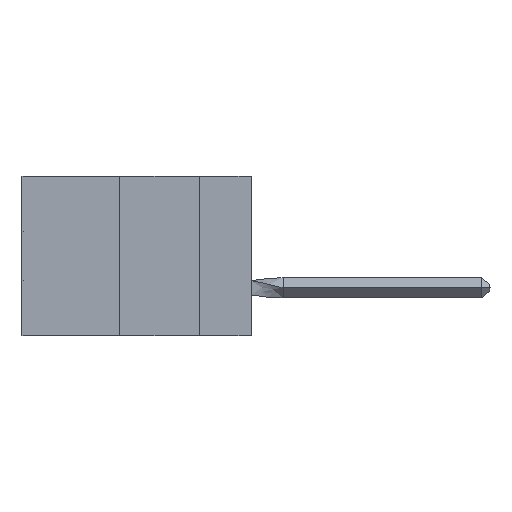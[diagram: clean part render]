
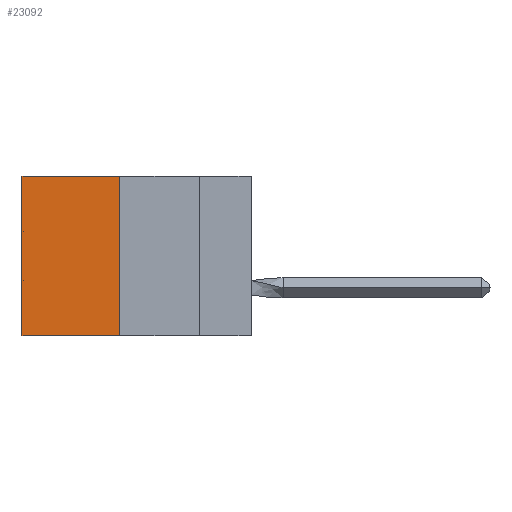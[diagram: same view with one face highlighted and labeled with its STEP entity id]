
A CAD part, left-side view. The second image highlights one B-rep face of the part: STEP entity #23092.
In plain terms, the highlighted planar face has unit normal (-1, 0, 0).
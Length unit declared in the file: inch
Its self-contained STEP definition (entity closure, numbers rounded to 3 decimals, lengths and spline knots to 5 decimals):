
#3802 = VECTOR ( 'NONE', #44119, 39.37008 ) ;
#6361 = VERTEX_POINT ( 'NONE', #9219 ) ;
#6470 = EDGE_CURVE ( 'NONE', #21489, #6361, #34841, .T. ) ;
#9219 = CARTESIAN_POINT ( 'NONE',  ( 0.305, 0.72, -0.5 ) ) ;
#9401 = EDGE_CURVE ( 'NONE', #30376, #21489, #21470, .T. ) ;
#9941 = FACE_OUTER_BOUND ( 'NONE', #44193, .T. ) ;
#12014 = DIRECTION ( 'NONE',  ( 0., 1., 0. ) ) ;
#12082 = VERTEX_POINT ( 'NONE', #38996 ) ;
#12298 = AXIS2_PLACEMENT_3D ( 'NONE', #26361, #12898, #33242 ) ;
#12898 = DIRECTION ( 'NONE',  ( 1., 0., 0. ) ) ;
#16788 = CARTESIAN_POINT ( 'NONE',  ( 0.305, 0.413, -0.5 ) ) ;
#17847 = ORIENTED_EDGE ( 'NONE', *, *, #36858, .T. ) ;
#18082 = CARTESIAN_POINT ( 'NONE',  ( 0.305, 0.413, 0. ) ) ;
#19926 = DIRECTION ( 'NONE',  ( 0., 0., -1. ) ) ;
#21470 = LINE ( 'NONE', #30815, #30567 ) ;
#21489 = VERTEX_POINT ( 'NONE', #39032 ) ;
#22206 = CARTESIAN_POINT ( 'NONE',  ( 0.305, 0.413, 0. ) ) ;
#23092 = ADVANCED_FACE ( 'NONE', ( #9941 ), #37121, .F. ) ;
#26361 = CARTESIAN_POINT ( 'NONE',  ( 0.305, 0.413, -0.5 ) ) ;
#27143 = ORIENTED_EDGE ( 'NONE', *, *, #35543, .T. ) ;
#27373 = LINE ( 'NONE', #22206, #38057 ) ;
#27498 = LINE ( 'NONE', #30596, #34481 ) ;
#28804 = ORIENTED_EDGE ( 'NONE', *, *, #9401, .F. ) ;
#30376 = VERTEX_POINT ( 'NONE', #18082 ) ;
#30567 = VECTOR ( 'NONE', #19926, 39.37008 ) ;
#30596 = CARTESIAN_POINT ( 'NONE',  ( 0.305, 0.72, -0.5 ) ) ;
#30815 = CARTESIAN_POINT ( 'NONE',  ( 0.305, 0.413, -0.5 ) ) ;
#33242 = DIRECTION ( 'NONE',  ( 0., 0., -1. ) ) ;
#34481 = VECTOR ( 'NONE', #43976, 39.37008 ) ;
#34539 = ORIENTED_EDGE ( 'NONE', *, *, #6470, .F. ) ;
#34841 = LINE ( 'NONE', #16788, #3802 ) ;
#35543 = EDGE_CURVE ( 'NONE', #12082, #6361, #27498, .T. ) ;
#36858 = EDGE_CURVE ( 'NONE', #30376, #12082, #27373, .T. ) ;
#37121 = PLANE ( 'NONE',  #12298 ) ;
#38057 = VECTOR ( 'NONE', #12014, 39.37008 ) ;
#38996 = CARTESIAN_POINT ( 'NONE',  ( 0.305, 0.72, 0. ) ) ;
#39032 = CARTESIAN_POINT ( 'NONE',  ( 0.305, 0.413, -0.5 ) ) ;
#43976 = DIRECTION ( 'NONE',  ( 0., 0., -1. ) ) ;
#44119 = DIRECTION ( 'NONE',  ( 0., 1., 0. ) ) ;
#44193 = EDGE_LOOP ( 'NONE', ( #27143, #34539, #28804, #17847 ) ) ;
